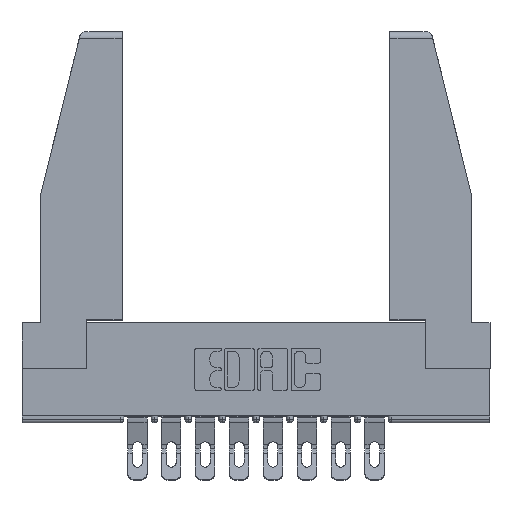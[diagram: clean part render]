
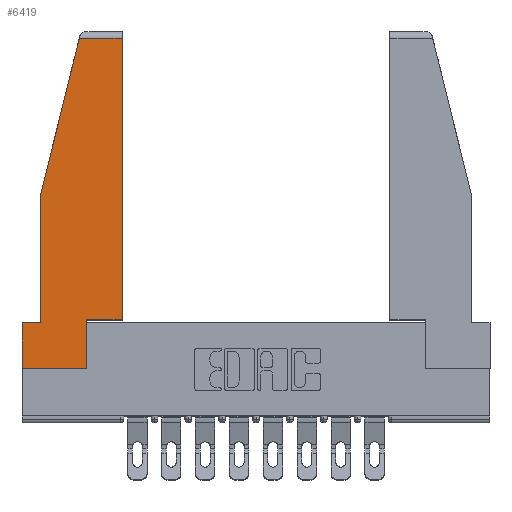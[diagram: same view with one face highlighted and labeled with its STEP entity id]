
A CAD part, top view. The second image highlights one B-rep face of the part: STEP entity #6419.
In plain terms, the highlighted planar face has unit normal (0, 0, 1).
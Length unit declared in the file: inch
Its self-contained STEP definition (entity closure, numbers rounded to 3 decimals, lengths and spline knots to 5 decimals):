
#317 = ORIENTED_EDGE ( 'NONE', *, *, #4773, .T. ) ;
#610 = VECTOR ( 'NONE', #4560, 39.37008 ) ;
#679 = LINE ( 'NONE', #10019, #2783 ) ;
#753 = CARTESIAN_POINT ( 'NONE',  ( 0., 0.21, 0. ) ) ;
#822 = LINE ( 'NONE', #13203, #610 ) ;
#1034 = DIRECTION ( 'NONE',  ( 1., 0., 0. ) ) ;
#1048 = LINE ( 'NONE', #753, #5857 ) ;
#1488 = CARTESIAN_POINT ( 'NONE',  ( 0., 0., 0. ) ) ;
#1657 = EDGE_CURVE ( 'NONE', #14033, #10159, #10528, .T. ) ;
#1914 = CARTESIAN_POINT ( 'NONE',  ( 0.461, 1.52, 0. ) ) ;
#2124 = DIRECTION ( 'NONE',  ( 1., 0., 0. ) ) ;
#2254 = CARTESIAN_POINT ( 'NONE',  ( 0.297, 0., 0. ) ) ;
#2390 = CARTESIAN_POINT ( 'NONE',  ( 0.271, 1.55, 0. ) ) ;
#2469 = ORIENTED_EDGE ( 'NONE', *, *, #13150, .T. ) ;
#2549 = AXIS2_PLACEMENT_3D ( 'NONE', #13105, #7065, #1034 ) ;
#2689 = VERTEX_POINT ( 'NONE', #10397 ) ;
#2783 = VECTOR ( 'NONE', #10071, 39.37008 ) ;
#2930 = FACE_OUTER_BOUND ( 'NONE', #5354, .T. ) ;
#2984 = CARTESIAN_POINT ( 'NONE',  ( 0.086, 0.8, 0. ) ) ;
#2991 = VECTOR ( 'NONE', #13726, 39.37008 ) ;
#3178 = DIRECTION ( 'NONE',  ( -1., 0., 0. ) ) ;
#4166 = DIRECTION ( 'NONE',  ( 0., 1., 0. ) ) ;
#4403 = ORIENTED_EDGE ( 'NONE', *, *, #12849, .T. ) ;
#4560 = DIRECTION ( 'NONE',  ( -1., 0., 0. ) ) ;
#4567 = PLANE ( 'NONE',  #2549 ) ;
#4765 = CARTESIAN_POINT ( 'NONE',  ( 0., 0., 0. ) ) ;
#4773 = EDGE_CURVE ( 'NONE', #9222, #14348, #14688, .T. ) ;
#5354 = EDGE_LOOP ( 'NONE', ( #317, #5430, #6827, #4403, #2469, #15835, #11697, #5820, #8807 ) ) ;
#5430 = ORIENTED_EDGE ( 'NONE', *, *, #14430, .T. ) ;
#5678 = LINE ( 'NONE', #10170, #13349 ) ;
#5820 = ORIENTED_EDGE ( 'NONE', *, *, #9277, .T. ) ;
#5857 = VECTOR ( 'NONE', #3178, 39.37008 ) ;
#5931 = VERTEX_POINT ( 'NONE', #2254 ) ;
#6191 = VERTEX_POINT ( 'NONE', #4765 ) ;
#6419 = ADVANCED_FACE ( 'NONE', ( #2930 ), #4567, .T. ) ;
#6528 = LINE ( 'NONE', #1488, #15713 ) ;
#6673 = CARTESIAN_POINT ( 'NONE',  ( 0.297, 0.223, 0. ) ) ;
#6827 = ORIENTED_EDGE ( 'NONE', *, *, #1657, .T. ) ;
#7065 = DIRECTION ( 'NONE',  ( 0., 0., 1. ) ) ;
#7219 = LINE ( 'NONE', #9486, #12759 ) ;
#7279 = VECTOR ( 'NONE', #4166, 39.37008 ) ;
#7288 = DIRECTION ( 'NONE',  ( -0.239, -0.971, 0. ) ) ;
#8142 = CARTESIAN_POINT ( 'NONE',  ( 0.461, 0.223, 0. ) ) ;
#8289 = EDGE_CURVE ( 'NONE', #6191, #5931, #6528, .T. ) ;
#8807 = ORIENTED_EDGE ( 'NONE', *, *, #12611, .T. ) ;
#8997 = LINE ( 'NONE', #9028, #7279 ) ;
#9028 = CARTESIAN_POINT ( 'NONE',  ( 0.297, 0., 0. ) ) ;
#9222 = VERTEX_POINT ( 'NONE', #8142 ) ;
#9277 = EDGE_CURVE ( 'NONE', #5931, #10184, #8997, .T. ) ;
#9486 = CARTESIAN_POINT ( 'NONE',  ( 0.297, 0.223, 0. ) ) ;
#10019 = CARTESIAN_POINT ( 'NONE',  ( 0.086, 0.8, 0. ) ) ;
#10048 = DIRECTION ( 'NONE',  ( 1., 0., 0. ) ) ;
#10071 = DIRECTION ( 'NONE',  ( 0., -1., 0. ) ) ;
#10159 = VERTEX_POINT ( 'NONE', #2984 ) ;
#10170 = CARTESIAN_POINT ( 'NONE',  ( 0., 0.21, 0. ) ) ;
#10184 = VERTEX_POINT ( 'NONE', #6673 ) ;
#10280 = DIRECTION ( 'NONE',  ( 0., -1., 0. ) ) ;
#10397 = CARTESIAN_POINT ( 'NONE',  ( 0.086, 0.21, 0. ) ) ;
#10528 = LINE ( 'NONE', #2390, #11494 ) ;
#11494 = VECTOR ( 'NONE', #7288, 39.37008 ) ;
#11697 = ORIENTED_EDGE ( 'NONE', *, *, #8289, .T. ) ;
#12468 = CARTESIAN_POINT ( 'NONE',  ( 0.2636, 1.52, 0. ) ) ;
#12611 = EDGE_CURVE ( 'NONE', #10184, #9222, #7219, .T. ) ;
#12759 = VECTOR ( 'NONE', #2124, 39.37008 ) ;
#12849 = EDGE_CURVE ( 'NONE', #10159, #2689, #679, .T. ) ;
#12893 = CARTESIAN_POINT ( 'NONE',  ( 0., 0.21, 0. ) ) ;
#13009 = EDGE_CURVE ( 'NONE', #15455, #6191, #5678, .T. ) ;
#13105 = CARTESIAN_POINT ( 'NONE',  ( 0., 0., 0. ) ) ;
#13150 = EDGE_CURVE ( 'NONE', #2689, #15455, #1048, .T. ) ;
#13203 = CARTESIAN_POINT ( 'NONE',  ( 0., 1.52, 0. ) ) ;
#13349 = VECTOR ( 'NONE', #10280, 39.37008 ) ;
#13726 = DIRECTION ( 'NONE',  ( 0., 1., 0. ) ) ;
#14033 = VERTEX_POINT ( 'NONE', #12468 ) ;
#14348 = VERTEX_POINT ( 'NONE', #1914 ) ;
#14430 = EDGE_CURVE ( 'NONE', #14348, #14033, #822, .T. ) ;
#14688 = LINE ( 'NONE', #15017, #2991 ) ;
#15017 = CARTESIAN_POINT ( 'NONE',  ( 0.461, 0.223, 0. ) ) ;
#15455 = VERTEX_POINT ( 'NONE', #12893 ) ;
#15713 = VECTOR ( 'NONE', #10048, 39.37008 ) ;
#15835 = ORIENTED_EDGE ( 'NONE', *, *, #13009, .T. ) ;
